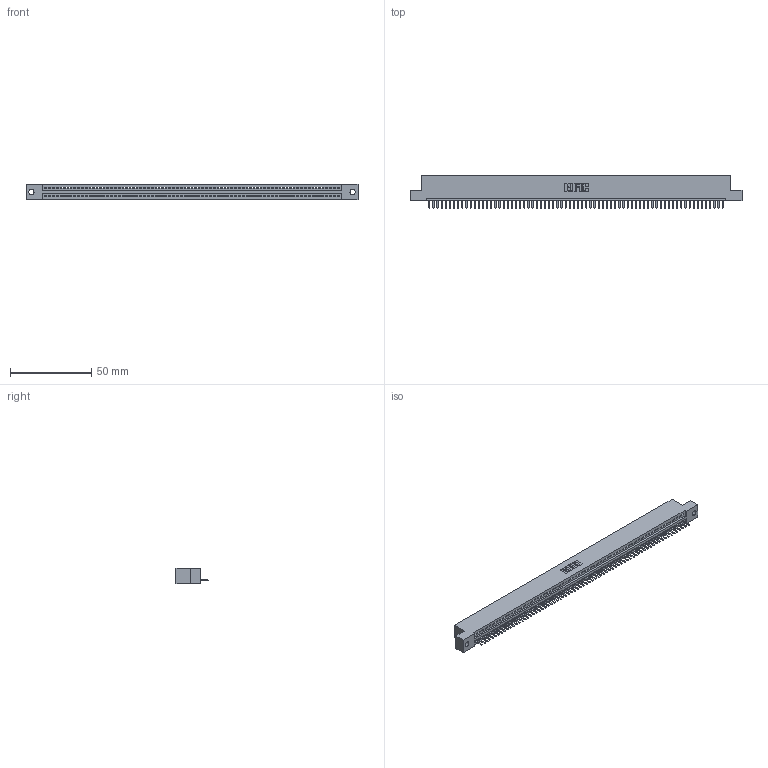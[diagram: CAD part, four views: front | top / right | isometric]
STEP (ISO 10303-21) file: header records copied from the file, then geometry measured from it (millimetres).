
FILE_DESCRIPTION (( 'STEP AP203' ), '1' );
FILE_NAME ('395-072-520-102.STEP', '2019-10-26T07:19:26', ( '' ), ( '' ), 'SwSTEP 2.0', 'SolidWorks 2016', '' );
FILE_SCHEMA (( 'CONFIG_CONTROL_DESIGN' ));
Length unit declared in the file: inch
Products named in the file (3): 345-292-001_345-293-120; 395-072-520-102; 345 Part_Flush Mounting Lugs - 0.128 Dia
Assembly tree (73 placements, depth 2):
  395-072-520-102
    345 Part_Flush Mounting Lugs - 0.128 Dia
    345-292-001_345-293-120  x72
Bounding box: 204.09 x 19.68 x 9.4 mm (x, y, z)
Volume: 19386.5 mm3; surface area: 25221.6 mm2
Topology: 73 solids, 73 shells, 4590 faces, 13589 edges, 8866 vertices
Faces by surface type: plane 3104, cylinder 1486
Entity records: 50267 total; most frequent: CARTESIAN_POINT 8724, ORIENTED_EDGE 8718, DIRECTION 7563, EDGE_CURVE 4359, VECTOR 3935, LINE 3935, VERTEX_POINT 2902, AXIS2_PLACEMENT_3D 1814
